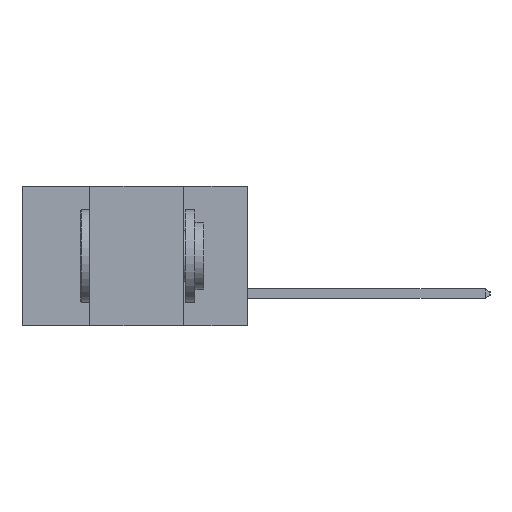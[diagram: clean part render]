
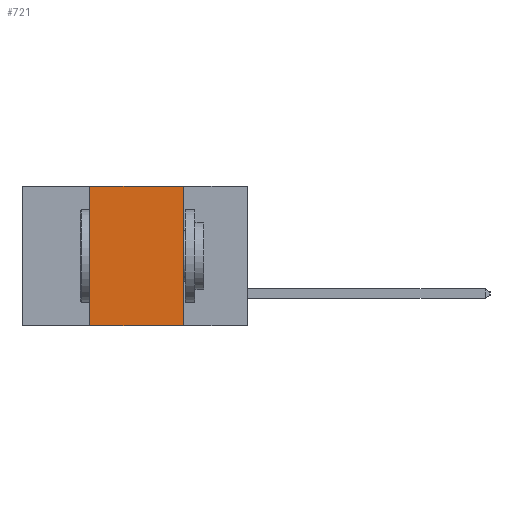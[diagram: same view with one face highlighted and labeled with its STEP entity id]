
A CAD part, left-side view. The second image highlights one B-rep face of the part: STEP entity #721.
In plain terms, the highlighted planar face has unit normal (-1, 0, 0).
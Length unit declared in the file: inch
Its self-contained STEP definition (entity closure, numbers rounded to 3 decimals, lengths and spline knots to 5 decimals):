
#721 = ADVANCED_FACE ( 'NONE', ( #4059 ), #12096, .F. ) ;
#728 = DIRECTION ( 'NONE',  ( 0., -1., 0. ) ) ;
#1036 = VERTEX_POINT ( 'NONE', #13902 ) ;
#1194 = VECTOR ( 'NONE', #728, 39.37008 ) ;
#1315 = CARTESIAN_POINT ( 'NONE',  ( 0., 0.17, -0.37 ) ) ;
#1577 = EDGE_CURVE ( 'NONE', #4471, #9452, #3324, .T. ) ;
#2304 = LINE ( 'NONE', #4937, #9710 ) ;
#2334 = DIRECTION ( 'NONE',  ( 0., 0., -1. ) ) ;
#2808 = CARTESIAN_POINT ( 'NONE',  ( 0., 0.17, -0.37 ) ) ;
#2870 = DIRECTION ( 'NONE',  ( 0., 0., -1. ) ) ;
#3324 = LINE ( 'NONE', #10067, #1194 ) ;
#3483 = ORIENTED_EDGE ( 'NONE', *, *, #4522, .F. ) ;
#3978 = CARTESIAN_POINT ( 'NONE',  ( 0., 0.6, 0. ) ) ;
#4059 = FACE_OUTER_BOUND ( 'NONE', #7771, .T. ) ;
#4471 = VERTEX_POINT ( 'NONE', #8963 ) ;
#4522 = EDGE_CURVE ( 'NONE', #1036, #9452, #8089, .T. ) ;
#4937 = CARTESIAN_POINT ( 'NONE',  ( 0., 0.6, 0. ) ) ;
#5904 = VECTOR ( 'NONE', #2334, 39.37008 ) ;
#7505 = EDGE_CURVE ( 'NONE', #7895, #1036, #2304, .T. ) ;
#7556 = ORIENTED_EDGE ( 'NONE', *, *, #1577, .T. ) ;
#7764 = CARTESIAN_POINT ( 'NONE',  ( 0., 0.42, -0.37 ) ) ;
#7771 = EDGE_LOOP ( 'NONE', ( #3483, #9986, #10956, #7556 ) ) ;
#7895 = VERTEX_POINT ( 'NONE', #10452 ) ;
#8089 = LINE ( 'NONE', #1315, #5904 ) ;
#8473 = VECTOR ( 'NONE', #12433, 39.37008 ) ;
#8786 = DIRECTION ( 'NONE',  ( 1., 0., 0. ) ) ;
#8963 = CARTESIAN_POINT ( 'NONE',  ( 0., 0.42, -0.37 ) ) ;
#9452 = VERTEX_POINT ( 'NONE', #2808 ) ;
#9494 = DIRECTION ( 'NONE',  ( 0., -1., 0. ) ) ;
#9710 = VECTOR ( 'NONE', #9494, 39.37008 ) ;
#9986 = ORIENTED_EDGE ( 'NONE', *, *, #7505, .F. ) ;
#10067 = CARTESIAN_POINT ( 'NONE',  ( 0., 0.6, -0.37 ) ) ;
#10452 = CARTESIAN_POINT ( 'NONE',  ( 0., 0.42, 0. ) ) ;
#10956 = ORIENTED_EDGE ( 'NONE', *, *, #11584, .F. ) ;
#11584 = EDGE_CURVE ( 'NONE', #4471, #7895, #11923, .T. ) ;
#11923 = LINE ( 'NONE', #7764, #8473 ) ;
#12096 = PLANE ( 'NONE',  #14832 ) ;
#12433 = DIRECTION ( 'NONE',  ( 0., 0., 1. ) ) ;
#13902 = CARTESIAN_POINT ( 'NONE',  ( 0., 0.17, 0. ) ) ;
#14832 = AXIS2_PLACEMENT_3D ( 'NONE', #3978, #8786, #2870 ) ;
